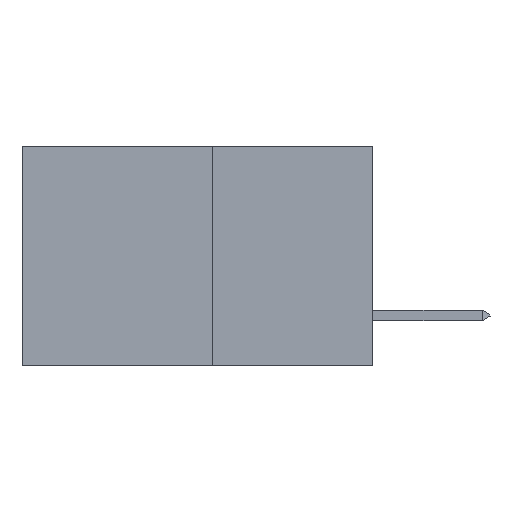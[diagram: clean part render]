
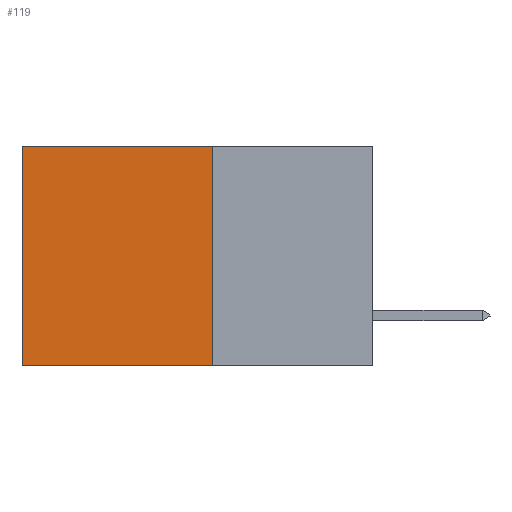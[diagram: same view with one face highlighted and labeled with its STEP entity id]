
A CAD part, left-side view. The second image highlights one B-rep face of the part: STEP entity #119.
In plain terms, the highlighted planar face has unit normal (-1, 0, 0).
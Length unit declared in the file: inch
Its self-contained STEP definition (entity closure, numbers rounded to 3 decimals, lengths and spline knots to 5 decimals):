
#119 = ADVANCED_FACE ( 'NONE', ( #3554 ), #14086, .F. ) ;
#312 = LINE ( 'NONE', #5372, #9086 ) ;
#930 = LINE ( 'NONE', #10768, #7718 ) ;
#1557 = ORIENTED_EDGE ( 'NONE', *, *, #11204, .T. ) ;
#1624 = VERTEX_POINT ( 'NONE', #4842 ) ;
#1948 = CARTESIAN_POINT ( 'NONE',  ( 0.277, 0.27, -0.37 ) ) ;
#3020 = EDGE_CURVE ( 'NONE', #12008, #1624, #930, .T. ) ;
#3021 = ORIENTED_EDGE ( 'NONE', *, *, #13361, .F. ) ;
#3150 = LINE ( 'NONE', #12095, #9180 ) ;
#3362 = ORIENTED_EDGE ( 'NONE', *, *, #3020, .F. ) ;
#3554 = FACE_OUTER_BOUND ( 'NONE', #10581, .T. ) ;
#4842 = CARTESIAN_POINT ( 'NONE',  ( 0.277, 0.59, -0.37 ) ) ;
#5372 = CARTESIAN_POINT ( 'NONE',  ( 0.277, 0.27, 0. ) ) ;
#6321 = LINE ( 'NONE', #10363, #14903 ) ;
#6616 = DIRECTION ( 'NONE',  ( 1., 0., 0. ) ) ;
#6620 = VERTEX_POINT ( 'NONE', #8232 ) ;
#7718 = VECTOR ( 'NONE', #12861, 39.37008 ) ;
#8232 = CARTESIAN_POINT ( 'NONE',  ( 0.277, 0.59, 0. ) ) ;
#8641 = AXIS2_PLACEMENT_3D ( 'NONE', #1948, #6616, #10950 ) ;
#9086 = VECTOR ( 'NONE', #11179, 39.37008 ) ;
#9180 = VECTOR ( 'NONE', #13208, 39.37008 ) ;
#9616 = CARTESIAN_POINT ( 'NONE',  ( 0.277, 0.27, 0. ) ) ;
#10144 = EDGE_CURVE ( 'NONE', #12069, #6620, #312, .T. ) ;
#10363 = CARTESIAN_POINT ( 'NONE',  ( 0.277, 0.59, -0.37 ) ) ;
#10581 = EDGE_LOOP ( 'NONE', ( #1557, #3362, #3021, #11785 ) ) ;
#10768 = CARTESIAN_POINT ( 'NONE',  ( 0.277, 0.27, -0.37 ) ) ;
#10950 = DIRECTION ( 'NONE',  ( 0., 0., -1. ) ) ;
#11179 = DIRECTION ( 'NONE',  ( 0., 1., 0. ) ) ;
#11204 = EDGE_CURVE ( 'NONE', #6620, #1624, #6321, .T. ) ;
#11785 = ORIENTED_EDGE ( 'NONE', *, *, #10144, .T. ) ;
#12008 = VERTEX_POINT ( 'NONE', #12909 ) ;
#12069 = VERTEX_POINT ( 'NONE', #9616 ) ;
#12095 = CARTESIAN_POINT ( 'NONE',  ( 0.277, 0.27, -0.37 ) ) ;
#12597 = DIRECTION ( 'NONE',  ( 0., 0., -1. ) ) ;
#12861 = DIRECTION ( 'NONE',  ( 0., 1., 0. ) ) ;
#12909 = CARTESIAN_POINT ( 'NONE',  ( 0.277, 0.27, -0.37 ) ) ;
#13208 = DIRECTION ( 'NONE',  ( 0., 0., -1. ) ) ;
#13361 = EDGE_CURVE ( 'NONE', #12069, #12008, #3150, .T. ) ;
#14086 = PLANE ( 'NONE',  #8641 ) ;
#14903 = VECTOR ( 'NONE', #12597, 39.37008 ) ;
